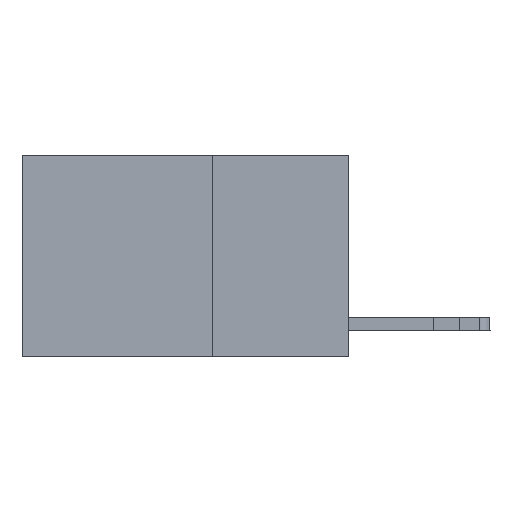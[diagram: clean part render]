
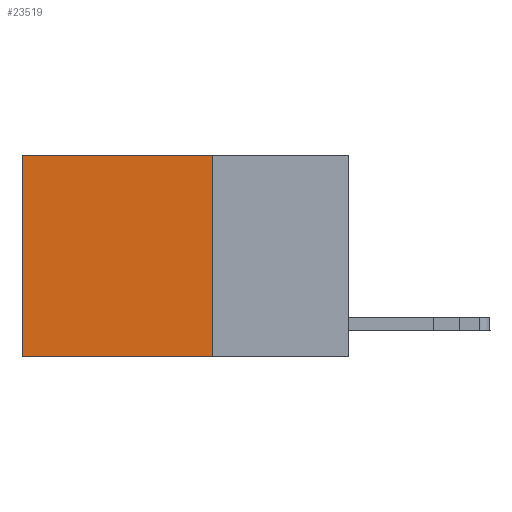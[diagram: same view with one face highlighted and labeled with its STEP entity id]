
A CAD part, left-side view. The second image highlights one B-rep face of the part: STEP entity #23519.
In plain terms, the highlighted planar face has unit normal (-1, 0, 0).
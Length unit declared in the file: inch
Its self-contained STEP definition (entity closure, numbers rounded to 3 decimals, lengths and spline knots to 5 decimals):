
#1792 = EDGE_CURVE ( 'NONE', #13061, #26388, #12317, .T. ) ;
#3474 = VECTOR ( 'NONE', #14280, 39.37008 ) ;
#4160 = CARTESIAN_POINT ( 'NONE',  ( 0.2625, 0.25, 0. ) ) ;
#4680 = AXIS2_PLACEMENT_3D ( 'NONE', #4160, #14472, #12328 ) ;
#5252 = EDGE_CURVE ( 'NONE', #5934, #15881, #26217, .T. ) ;
#5424 = EDGE_CURVE ( 'NONE', #13061, #5934, #10704, .T. ) ;
#5934 = VERTEX_POINT ( 'NONE', #19207 ) ;
#6410 = VECTOR ( 'NONE', #8052, 39.37008 ) ;
#6696 = EDGE_CURVE ( 'NONE', #26388, #15881, #16469, .T. ) ;
#7073 = ORIENTED_EDGE ( 'NONE', *, *, #5252, .T. ) ;
#7693 = ORIENTED_EDGE ( 'NONE', *, *, #1792, .F. ) ;
#8052 = DIRECTION ( 'NONE',  ( 0., 0., -1. ) ) ;
#9209 = ORIENTED_EDGE ( 'NONE', *, *, #6696, .F. ) ;
#10072 = PLANE ( 'NONE',  #4680 ) ;
#10704 = LINE ( 'NONE', #24329, #18330 ) ;
#11477 = ORIENTED_EDGE ( 'NONE', *, *, #5424, .T. ) ;
#12317 = LINE ( 'NONE', #12724, #6410 ) ;
#12328 = DIRECTION ( 'NONE',  ( 0., 0., -1. ) ) ;
#12724 = CARTESIAN_POINT ( 'NONE',  ( 0.2625, 0.25, 0. ) ) ;
#13061 = VERTEX_POINT ( 'NONE', #20598 ) ;
#14280 = DIRECTION ( 'NONE',  ( 0., 1., 0. ) ) ;
#14321 = DIRECTION ( 'NONE',  ( 0., 1., 0. ) ) ;
#14450 = CARTESIAN_POINT ( 'NONE',  ( 0.2625, 0.25, -0.37 ) ) ;
#14472 = DIRECTION ( 'NONE',  ( 1., 0., 0. ) ) ;
#15881 = VERTEX_POINT ( 'NONE', #19495 ) ;
#16469 = LINE ( 'NONE', #14450, #3474 ) ;
#17106 = VECTOR ( 'NONE', #17808, 39.37008 ) ;
#17808 = DIRECTION ( 'NONE',  ( 0., 0., -1. ) ) ;
#18330 = VECTOR ( 'NONE', #14321, 39.37008 ) ;
#19207 = CARTESIAN_POINT ( 'NONE',  ( 0.2625, 0.6, 0. ) ) ;
#19495 = CARTESIAN_POINT ( 'NONE',  ( 0.2625, 0.6, -0.37 ) ) ;
#19676 = CARTESIAN_POINT ( 'NONE',  ( 0.2625, 0.25, -0.37 ) ) ;
#20598 = CARTESIAN_POINT ( 'NONE',  ( 0.2625, 0.25, 0. ) ) ;
#20608 = FACE_OUTER_BOUND ( 'NONE', #25899, .T. ) ;
#22055 = CARTESIAN_POINT ( 'NONE',  ( 0.2625, 0.6, 0. ) ) ;
#23519 = ADVANCED_FACE ( 'NONE', ( #20608 ), #10072, .F. ) ;
#24329 = CARTESIAN_POINT ( 'NONE',  ( 0.2625, 0.25, 0. ) ) ;
#25899 = EDGE_LOOP ( 'NONE', ( #7073, #9209, #7693, #11477 ) ) ;
#26217 = LINE ( 'NONE', #22055, #17106 ) ;
#26388 = VERTEX_POINT ( 'NONE', #19676 ) ;
